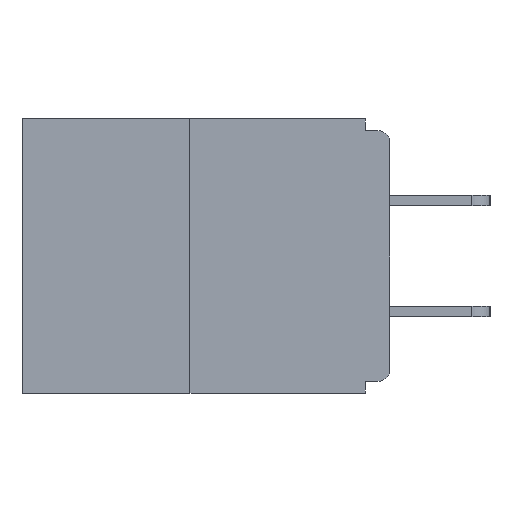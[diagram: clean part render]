
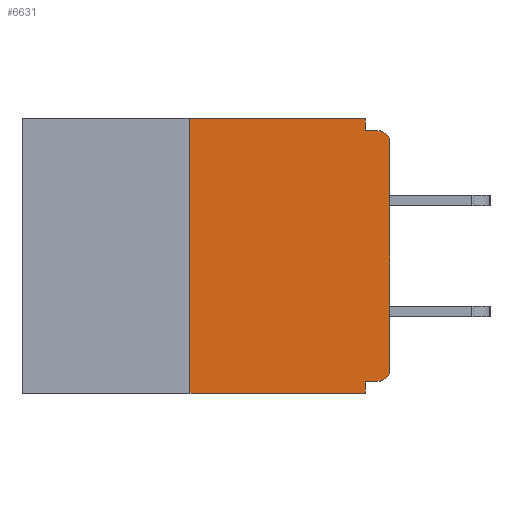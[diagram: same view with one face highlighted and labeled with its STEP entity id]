
A CAD part, left-side view. The second image highlights one B-rep face of the part: STEP entity #6631.
In plain terms, the highlighted planar face has unit normal (-1, 0, 0).
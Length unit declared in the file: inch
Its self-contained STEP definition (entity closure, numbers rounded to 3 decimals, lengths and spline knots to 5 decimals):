
#37 = VECTOR ( 'NONE', #11671, 39.37008 ) ;
#78 = CARTESIAN_POINT ( 'NONE',  ( 0., 0., 0. ) ) ;
#368 = EDGE_CURVE ( 'NONE', #11160, #13870, #9815, .T. ) ;
#493 = EDGE_CURVE ( 'NONE', #11160, #5764, #12621, .T. ) ;
#946 = LINE ( 'NONE', #4672, #9117 ) ;
#959 = EDGE_CURVE ( 'NONE', #7484, #9650, #11483, .T. ) ;
#977 = AXIS2_PLACEMENT_3D ( 'NONE', #13735, #1018, #13659 ) ;
#1018 = DIRECTION ( 'NONE',  ( -1., 0., 0. ) ) ;
#1022 = VECTOR ( 'NONE', #10090, 39.37008 ) ;
#1235 = EDGE_CURVE ( 'NONE', #5061, #7484, #3501, .T. ) ;
#1680 = VECTOR ( 'NONE', #12546, 39.37008 ) ;
#1752 = ORIENTED_EDGE ( 'NONE', *, *, #6828, .F. ) ;
#1797 = AXIS2_PLACEMENT_3D ( 'NONE', #2732, #7234, #12044 ) ;
#2002 = LINE ( 'NONE', #10165, #1022 ) ;
#2012 = CARTESIAN_POINT ( 'NONE',  ( 0., 0.031, -0.328 ) ) ;
#2170 = CARTESIAN_POINT ( 'NONE',  ( 0., 0.031, -0.343 ) ) ;
#2385 = VERTEX_POINT ( 'NONE', #8757 ) ;
#2732 = CARTESIAN_POINT ( 'NONE',  ( 0., 0.015, -0.313 ) ) ;
#2857 = LINE ( 'NONE', #11113, #3963 ) ;
#3067 = CARTESIAN_POINT ( 'NONE',  ( 0., 0.015, -0.015 ) ) ;
#3208 = DIRECTION ( 'NONE',  ( 0., 0., -1. ) ) ;
#3342 = ORIENTED_EDGE ( 'NONE', *, *, #7624, .T. ) ;
#3467 = CARTESIAN_POINT ( 'NONE',  ( 0., 0.015, -0.328 ) ) ;
#3501 = LINE ( 'NONE', #78, #7058 ) ;
#3963 = VECTOR ( 'NONE', #10045, 39.37008 ) ;
#4298 = EDGE_CURVE ( 'NONE', #13870, #5728, #13106, .T. ) ;
#4490 = PLANE ( 'NONE',  #14417 ) ;
#4672 = CARTESIAN_POINT ( 'NONE',  ( 0., 0., -0.328 ) ) ;
#4730 = CARTESIAN_POINT ( 'NONE',  ( 0., 0.25, -0.343 ) ) ;
#4923 = EDGE_CURVE ( 'NONE', #12494, #5764, #11415, .T. ) ;
#5061 = VERTEX_POINT ( 'NONE', #5115 ) ;
#5115 = CARTESIAN_POINT ( 'NONE',  ( 0., 0., -0.313 ) ) ;
#5485 = CARTESIAN_POINT ( 'NONE',  ( 0., 0.46, 0. ) ) ;
#5663 = VERTEX_POINT ( 'NONE', #3467 ) ;
#5687 = CIRCLE ( 'NONE', #1797, 0.015 ) ;
#5728 = VERTEX_POINT ( 'NONE', #15032 ) ;
#5764 = VERTEX_POINT ( 'NONE', #2170 ) ;
#6631 = ADVANCED_FACE ( 'NONE', ( #11298 ), #4490, .F. ) ;
#6828 = EDGE_CURVE ( 'NONE', #5728, #2385, #2857, .T. ) ;
#7008 = CARTESIAN_POINT ( 'NONE',  ( 0., 0.46, 0. ) ) ;
#7058 = VECTOR ( 'NONE', #8137, 39.37008 ) ;
#7234 = DIRECTION ( 'NONE',  ( -1., 0., 0. ) ) ;
#7484 = VERTEX_POINT ( 'NONE', #8144 ) ;
#7624 = EDGE_CURVE ( 'NONE', #5663, #5061, #5687, .T. ) ;
#7826 = ORIENTED_EDGE ( 'NONE', *, *, #493, .T. ) ;
#8137 = DIRECTION ( 'NONE',  ( 0., 0., 1. ) ) ;
#8144 = CARTESIAN_POINT ( 'NONE',  ( 0., 0., -0.03 ) ) ;
#8248 = ORIENTED_EDGE ( 'NONE', *, *, #14630, .F. ) ;
#8550 = ORIENTED_EDGE ( 'NONE', *, *, #959, .T. ) ;
#8723 = CARTESIAN_POINT ( 'NONE',  ( 0., 0.25, 0. ) ) ;
#8757 = CARTESIAN_POINT ( 'NONE',  ( 0., 0.031, -0.015 ) ) ;
#8783 = EDGE_CURVE ( 'NONE', #5663, #12494, #946, .T. ) ;
#8884 = CARTESIAN_POINT ( 'NONE',  ( 0., 0.031, -0.343 ) ) ;
#8989 = DIRECTION ( 'NONE',  ( 1., 0., 0. ) ) ;
#9039 = CARTESIAN_POINT ( 'NONE',  ( 0., 0.46, -0.343 ) ) ;
#9117 = VECTOR ( 'NONE', #10321, 39.37008 ) ;
#9238 = VECTOR ( 'NONE', #11117, 39.37008 ) ;
#9564 = ORIENTED_EDGE ( 'NONE', *, *, #1235, .T. ) ;
#9650 = VERTEX_POINT ( 'NONE', #3067 ) ;
#9775 = ORIENTED_EDGE ( 'NONE', *, *, #4923, .F. ) ;
#9815 = LINE ( 'NONE', #8723, #9238 ) ;
#10045 = DIRECTION ( 'NONE',  ( 0., 0., -1. ) ) ;
#10090 = DIRECTION ( 'NONE',  ( 0., -1., 0. ) ) ;
#10165 = CARTESIAN_POINT ( 'NONE',  ( 0., 0., -0.015 ) ) ;
#10321 = DIRECTION ( 'NONE',  ( 0., 1., 0. ) ) ;
#10338 = DIRECTION ( 'NONE',  ( 0., 0., -1. ) ) ;
#11113 = CARTESIAN_POINT ( 'NONE',  ( 0., 0.031, 0. ) ) ;
#11117 = DIRECTION ( 'NONE',  ( 0., 0., 1. ) ) ;
#11160 = VERTEX_POINT ( 'NONE', #4730 ) ;
#11298 = FACE_OUTER_BOUND ( 'NONE', #13085, .T. ) ;
#11361 = CARTESIAN_POINT ( 'NONE',  ( 0., 0.25, 0. ) ) ;
#11415 = LINE ( 'NONE', #8884, #12448 ) ;
#11420 = ORIENTED_EDGE ( 'NONE', *, *, #368, .F. ) ;
#11483 = CIRCLE ( 'NONE', #977, 0.015 ) ;
#11671 = DIRECTION ( 'NONE',  ( 0., -1., 0. ) ) ;
#12044 = DIRECTION ( 'NONE',  ( 0., 0., -1. ) ) ;
#12448 = VECTOR ( 'NONE', #10338, 39.37008 ) ;
#12494 = VERTEX_POINT ( 'NONE', #2012 ) ;
#12546 = DIRECTION ( 'NONE',  ( 0., -1., 0. ) ) ;
#12621 = LINE ( 'NONE', #9039, #1680 ) ;
#12807 = ORIENTED_EDGE ( 'NONE', *, *, #4298, .F. ) ;
#13085 = EDGE_LOOP ( 'NONE', ( #12807, #11420, #7826, #9775, #14044, #3342, #9564, #8550, #8248, #1752 ) ) ;
#13106 = LINE ( 'NONE', #7008, #37 ) ;
#13659 = DIRECTION ( 'NONE',  ( 0., 0., -1. ) ) ;
#13735 = CARTESIAN_POINT ( 'NONE',  ( 0., 0.015, -0.03 ) ) ;
#13870 = VERTEX_POINT ( 'NONE', #11361 ) ;
#14044 = ORIENTED_EDGE ( 'NONE', *, *, #8783, .F. ) ;
#14417 = AXIS2_PLACEMENT_3D ( 'NONE', #5485, #8989, #3208 ) ;
#14630 = EDGE_CURVE ( 'NONE', #2385, #9650, #2002, .T. ) ;
#15032 = CARTESIAN_POINT ( 'NONE',  ( 0., 0.031, 0. ) ) ;
